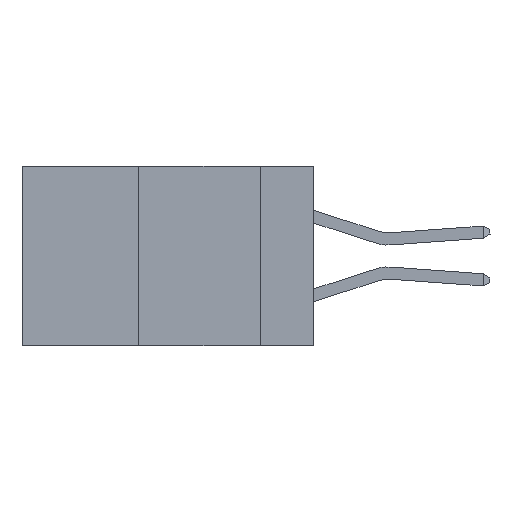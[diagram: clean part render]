
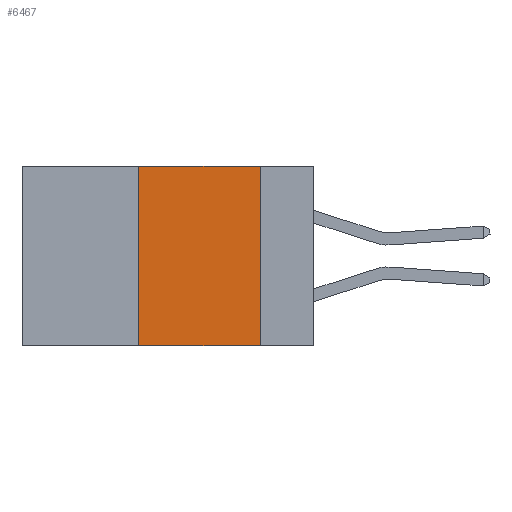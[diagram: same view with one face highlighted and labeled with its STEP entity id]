
A CAD part, left-side view. The second image highlights one B-rep face of the part: STEP entity #6467.
In plain terms, the highlighted planar face has unit normal (-1, 0, 0).
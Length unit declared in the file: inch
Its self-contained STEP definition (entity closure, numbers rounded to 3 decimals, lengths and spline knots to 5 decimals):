
#18 = VECTOR ( 'NONE', #20290, 39.37008 ) ;
#51 = EDGE_CURVE ( 'NONE', #2983, #22865, #18465, .T. ) ;
#189 = ORIENTED_EDGE ( 'NONE', *, *, #1735, .T. ) ;
#1735 = EDGE_CURVE ( 'NONE', #15495, #22865, #5910, .T. ) ;
#2752 = CARTESIAN_POINT ( 'NONE',  ( 0., 0.36, 0. ) ) ;
#2983 = VERTEX_POINT ( 'NONE', #7668 ) ;
#3482 = DIRECTION ( 'NONE',  ( 0., -1., 0. ) ) ;
#5098 = EDGE_LOOP ( 'NONE', ( #8009, #27294, #22971, #189 ) ) ;
#5290 = PLANE ( 'NONE',  #19140 ) ;
#5880 = DIRECTION ( 'NONE',  ( 0., 0., 1. ) ) ;
#5910 = LINE ( 'NONE', #22426, #18 ) ;
#6467 = ADVANCED_FACE ( 'NONE', ( #20310 ), #5290, .F. ) ;
#6708 = VECTOR ( 'NONE', #18179, 39.37008 ) ;
#7668 = CARTESIAN_POINT ( 'NONE',  ( 0., 0.11, 0. ) ) ;
#8009 = ORIENTED_EDGE ( 'NONE', *, *, #51, .F. ) ;
#8862 = VERTEX_POINT ( 'NONE', #2752 ) ;
#9105 = VECTOR ( 'NONE', #3482, 39.37008 ) ;
#9427 = EDGE_CURVE ( 'NONE', #8862, #2983, #20856, .T. ) ;
#13740 = CARTESIAN_POINT ( 'NONE',  ( 0., 0.11, 0. ) ) ;
#15495 = VERTEX_POINT ( 'NONE', #16381 ) ;
#16381 = CARTESIAN_POINT ( 'NONE',  ( 0., 0.36, -0.37 ) ) ;
#16489 = DIRECTION ( 'NONE',  ( 1., 0., 0. ) ) ;
#18179 = DIRECTION ( 'NONE',  ( 0., 0., -1. ) ) ;
#18465 = LINE ( 'NONE', #13740, #6708 ) ;
#19140 = AXIS2_PLACEMENT_3D ( 'NONE', #27178, #16489, #20668 ) ;
#20290 = DIRECTION ( 'NONE',  ( 0., -1., 0. ) ) ;
#20310 = FACE_OUTER_BOUND ( 'NONE', #5098, .T. ) ;
#20605 = EDGE_CURVE ( 'NONE', #15495, #8862, #27402, .T. ) ;
#20668 = DIRECTION ( 'NONE',  ( 0., 0., -1. ) ) ;
#20856 = LINE ( 'NONE', #20926, #9105 ) ;
#20926 = CARTESIAN_POINT ( 'NONE',  ( 0., 0.6, 0. ) ) ;
#22426 = CARTESIAN_POINT ( 'NONE',  ( 0., 0.6, -0.37 ) ) ;
#22747 = CARTESIAN_POINT ( 'NONE',  ( 0., 0.11, -0.37 ) ) ;
#22865 = VERTEX_POINT ( 'NONE', #22747 ) ;
#22971 = ORIENTED_EDGE ( 'NONE', *, *, #20605, .F. ) ;
#23111 = CARTESIAN_POINT ( 'NONE',  ( 0., 0.36, 0. ) ) ;
#24620 = VECTOR ( 'NONE', #5880, 39.37008 ) ;
#27178 = CARTESIAN_POINT ( 'NONE',  ( 0., 0.6, 0. ) ) ;
#27294 = ORIENTED_EDGE ( 'NONE', *, *, #9427, .F. ) ;
#27402 = LINE ( 'NONE', #23111, #24620 ) ;
